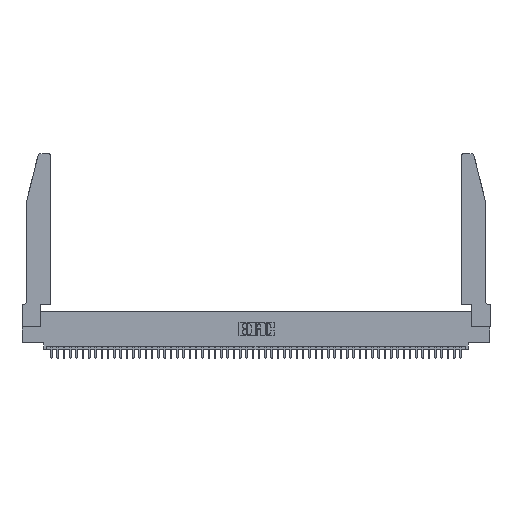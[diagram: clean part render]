
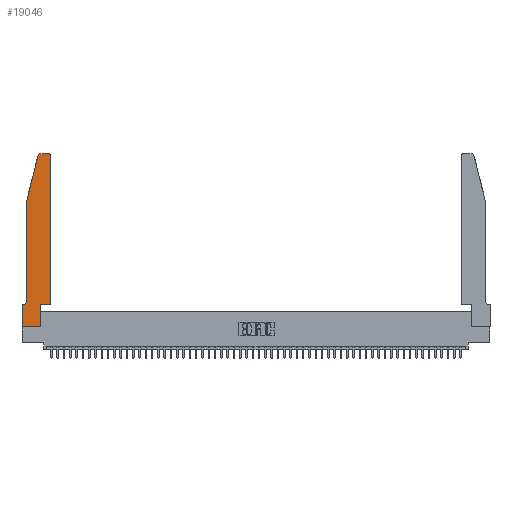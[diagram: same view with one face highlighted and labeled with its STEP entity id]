
A CAD part, top view. The second image highlights one B-rep face of the part: STEP entity #19046.
In plain terms, the highlighted planar face has unit normal (0, 0, 1).
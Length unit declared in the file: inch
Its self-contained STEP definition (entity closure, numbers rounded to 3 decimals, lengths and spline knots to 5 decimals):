
#594 = VECTOR ( 'NONE', #39229, 39.37008 ) ;
#1221 = CARTESIAN_POINT ( 'NONE',  ( 0.4205, 2.75, 0.37 ) ) ;
#1756 = DIRECTION ( 'NONE',  ( -1., 0., 0. ) ) ;
#1996 = DIRECTION ( 'NONE',  ( -1., 0., 0. ) ) ;
#2881 = DIRECTION ( 'NONE',  ( 0., -1., 0. ) ) ;
#3169 = EDGE_CURVE ( 'NONE', #43188, #36779, #51806, .T. ) ;
#4783 = VERTEX_POINT ( 'NONE', #27438 ) ;
#5557 = CARTESIAN_POINT ( 'NONE',  ( 0.284, 2.75, 0.37 ) ) ;
#6082 = ORIENTED_EDGE ( 'NONE', *, *, #46164, .T. ) ;
#6772 = LINE ( 'NONE', #9782, #48011 ) ;
#6981 = VERTEX_POINT ( 'NONE', #13764 ) ;
#7285 = ORIENTED_EDGE ( 'NONE', *, *, #41272, .T. ) ;
#7336 = AXIS2_PLACEMENT_3D ( 'NONE', #51406, #26938, #1996 ) ;
#7698 = CARTESIAN_POINT ( 'NONE',  ( 0., 0., 0.37 ) ) ;
#8145 = VERTEX_POINT ( 'NONE', #50868 ) ;
#8572 = CARTESIAN_POINT ( 'NONE',  ( 0.2865, 0.35, 0.37 ) ) ;
#9090 = CARTESIAN_POINT ( 'NONE',  ( 0.284, 2.72, 0.37 ) ) ;
#9782 = CARTESIAN_POINT ( 'NONE',  ( 0.0755, 2., 0.37 ) ) ;
#10059 = CARTESIAN_POINT ( 'NONE',  ( 0.2605, 2.75, 0.37 ) ) ;
#11736 = LINE ( 'NONE', #47835, #32337 ) ;
#11925 = DIRECTION ( 'NONE',  ( 0., -1., 0. ) ) ;
#11941 = ORIENTED_EDGE ( 'NONE', *, *, #17192, .T. ) ;
#12230 = VERTEX_POINT ( 'NONE', #35693 ) ;
#13094 = CIRCLE ( 'NONE', #31422, 0.03 ) ;
#13311 = DIRECTION ( 'NONE',  ( 1., 0., 0. ) ) ;
#13343 = AXIS2_PLACEMENT_3D ( 'NONE', #15036, #47852, #23350 ) ;
#13764 = CARTESIAN_POINT ( 'NONE',  ( 0., 0., 0.37 ) ) ;
#14765 = EDGE_CURVE ( 'NONE', #47355, #4783, #11736, .T. ) ;
#15036 = CARTESIAN_POINT ( 'NONE',  ( 0., 0.35, 0.37 ) ) ;
#15645 = CARTESIAN_POINT ( 'NONE',  ( 0.4505, 0.35, 0.37 ) ) ;
#15991 = ORIENTED_EDGE ( 'NONE', *, *, #24364, .T. ) ;
#16433 = CARTESIAN_POINT ( 'NONE',  ( 0.4205, 2.72, 0.37 ) ) ;
#16554 = ORIENTED_EDGE ( 'NONE', *, *, #22768, .T. ) ;
#17078 = ORIENTED_EDGE ( 'NONE', *, *, #22861, .T. ) ;
#17130 = ORIENTED_EDGE ( 'NONE', *, *, #3169, .T. ) ;
#17192 = EDGE_CURVE ( 'NONE', #8145, #43188, #50701, .T. ) ;
#18861 = CARTESIAN_POINT ( 'NONE',  ( 0.4505, 2.72, 0.37 ) ) ;
#19046 = ADVANCED_FACE ( 'NONE', ( #22466 ), #19228, .T. ) ;
#19228 = PLANE ( 'NONE',  #13343 ) ;
#20120 = VECTOR ( 'NONE', #11925, 39.37008 ) ;
#20588 = DIRECTION ( 'NONE',  ( 1., 0., 0. ) ) ;
#21391 = LINE ( 'NONE', #7698, #20120 ) ;
#22180 = VERTEX_POINT ( 'NONE', #18861 ) ;
#22205 = ORIENTED_EDGE ( 'NONE', *, *, #14765, .T. ) ;
#22258 = ORIENTED_EDGE ( 'NONE', *, *, #49942, .T. ) ;
#22335 = CARTESIAN_POINT ( 'NONE',  ( 0.0055, 0.35, 0.37 ) ) ;
#22466 = FACE_OUTER_BOUND ( 'NONE', #24613, .T. ) ;
#22768 = EDGE_CURVE ( 'NONE', #12230, #8145, #26534, .T. ) ;
#22835 = ORIENTED_EDGE ( 'NONE', *, *, #30359, .T. ) ;
#22861 = EDGE_CURVE ( 'NONE', #36779, #6981, #21391, .T. ) ;
#23140 = CIRCLE ( 'NONE', #28364, 0.03 ) ;
#23350 = DIRECTION ( 'NONE',  ( 1., 0., 0. ) ) ;
#24128 = VECTOR ( 'NONE', #49050, 39.37008 ) ;
#24364 = EDGE_CURVE ( 'NONE', #52964, #48930, #23140, .T. ) ;
#24613 = EDGE_LOOP ( 'NONE', ( #6082, #15991, #33245, #16554, #11941, #17130, #17078, #22258, #7285, #22205, #22835, #43983 ) ) ;
#25243 = VECTOR ( 'NONE', #2881, 39.37008 ) ;
#25392 = LINE ( 'NONE', #36678, #24128 ) ;
#26150 = CARTESIAN_POINT ( 'NONE',  ( 0.0755, 0.35, 0.37 ) ) ;
#26187 = CARTESIAN_POINT ( 'NONE',  ( 0.2865, 0., 0.37 ) ) ;
#26534 = LINE ( 'NONE', #48183, #25243 ) ;
#26938 = DIRECTION ( 'NONE',  ( 0., 0., -1. ) ) ;
#27438 = CARTESIAN_POINT ( 'NONE',  ( 0.4505, 0.35, 0.37 ) ) ;
#27647 = VECTOR ( 'NONE', #1756, 39.37008 ) ;
#28364 = AXIS2_PLACEMENT_3D ( 'NONE', #9090, #37889, #13311 ) ;
#29628 = LINE ( 'NONE', #15645, #39187 ) ;
#30228 = DIRECTION ( 'NONE',  ( -1., 0., 0. ) ) ;
#30359 = EDGE_CURVE ( 'NONE', #4783, #22180, #29628, .T. ) ;
#31422 = AXIS2_PLACEMENT_3D ( 'NONE', #16433, #45095, #20588 ) ;
#31986 = DIRECTION ( 'NONE',  ( 0., 1., 0. ) ) ;
#32337 = VECTOR ( 'NONE', #39562, 39.37008 ) ;
#33245 = ORIENTED_EDGE ( 'NONE', *, *, #40242, .T. ) ;
#33712 = LINE ( 'NONE', #35156, #594 ) ;
#35156 = CARTESIAN_POINT ( 'NONE',  ( 0.2865, 0.35, 0.37 ) ) ;
#35574 = CARTESIAN_POINT ( 'NONE',  ( 0.25487, 2.72718, 0.37 ) ) ;
#35693 = CARTESIAN_POINT ( 'NONE',  ( 0.0755, 2., 0.37 ) ) ;
#36516 = VERTEX_POINT ( 'NONE', #26187 ) ;
#36520 = VERTEX_POINT ( 'NONE', #1221 ) ;
#36678 = CARTESIAN_POINT ( 'NONE',  ( 0., 0., 0.37 ) ) ;
#36779 = VERTEX_POINT ( 'NONE', #52438 ) ;
#37889 = DIRECTION ( 'NONE',  ( 0., 0., 1. ) ) ;
#38467 = LINE ( 'NONE', #10059, #27647 ) ;
#39187 = VECTOR ( 'NONE', #31986, 39.37008 ) ;
#39229 = DIRECTION ( 'NONE',  ( 0., 1., 0. ) ) ;
#39562 = DIRECTION ( 'NONE',  ( 1., 0., 0. ) ) ;
#40242 = EDGE_CURVE ( 'NONE', #48930, #12230, #6772, .T. ) ;
#40882 = VECTOR ( 'NONE', #30228, 39.37008 ) ;
#41272 = EDGE_CURVE ( 'NONE', #36516, #47355, #33712, .T. ) ;
#43188 = VERTEX_POINT ( 'NONE', #22335 ) ;
#43983 = ORIENTED_EDGE ( 'NONE', *, *, #49951, .T. ) ;
#45095 = DIRECTION ( 'NONE',  ( 0., 0., 1. ) ) ;
#46164 = EDGE_CURVE ( 'NONE', #36520, #52964, #38467, .T. ) ;
#47355 = VERTEX_POINT ( 'NONE', #8572 ) ;
#47835 = CARTESIAN_POINT ( 'NONE',  ( 0.4505, 0.35, 0.37 ) ) ;
#47852 = DIRECTION ( 'NONE',  ( 0., 0., 1. ) ) ;
#48011 = VECTOR ( 'NONE', #50917, 39.37008 ) ;
#48183 = CARTESIAN_POINT ( 'NONE',  ( 0.0755, 2., 0.37 ) ) ;
#48930 = VERTEX_POINT ( 'NONE', #35574 ) ;
#49050 = DIRECTION ( 'NONE',  ( 1., 0., 0. ) ) ;
#49942 = EDGE_CURVE ( 'NONE', #6981, #36516, #25392, .T. ) ;
#49951 = EDGE_CURVE ( 'NONE', #22180, #36520, #13094, .T. ) ;
#50701 = CIRCLE ( 'NONE', #7336, 0.07 ) ;
#50868 = CARTESIAN_POINT ( 'NONE',  ( 0.0755, 0.42, 0.37 ) ) ;
#50917 = DIRECTION ( 'NONE',  ( -0.239, -0.971, 0. ) ) ;
#51406 = CARTESIAN_POINT ( 'NONE',  ( 0.0055, 0.42, 0.37 ) ) ;
#51806 = LINE ( 'NONE', #26150, #40882 ) ;
#52438 = CARTESIAN_POINT ( 'NONE',  ( 0., 0.35, 0.37 ) ) ;
#52964 = VERTEX_POINT ( 'NONE', #5557 ) ;
